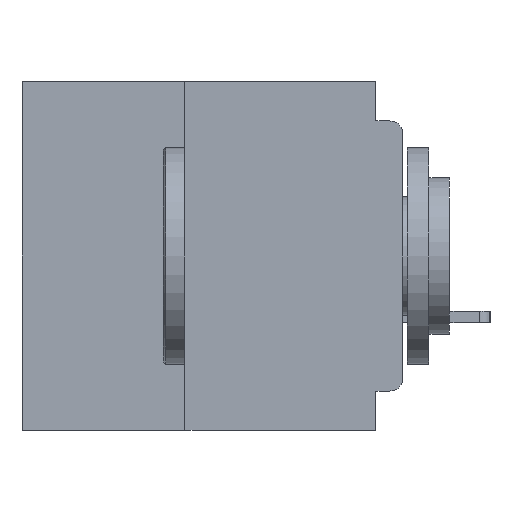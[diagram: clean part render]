
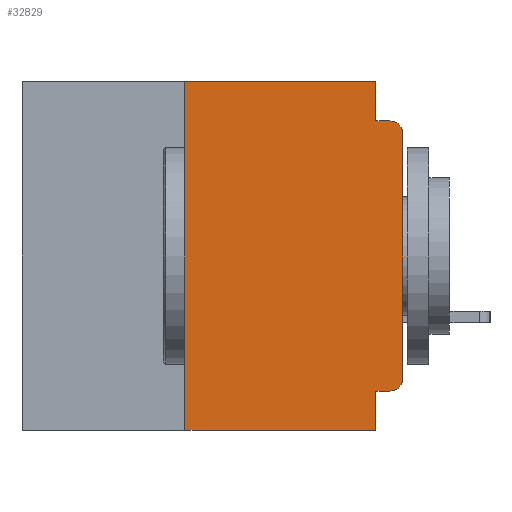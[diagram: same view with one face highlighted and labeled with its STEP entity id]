
A CAD part, left-side view. The second image highlights one B-rep face of the part: STEP entity #32829.
In plain terms, the highlighted planar face has unit normal (-1, 0, 0).
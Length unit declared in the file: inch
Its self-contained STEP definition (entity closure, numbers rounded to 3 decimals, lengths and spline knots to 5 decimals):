
#755 = EDGE_CURVE ( 'NONE', #26749, #22927, #27107, .T. ) ;
#1217 = VERTEX_POINT ( 'NONE', #17277 ) ;
#2097 = CARTESIAN_POINT ( 'NONE',  ( 0., 0.25, -0.4 ) ) ;
#2519 = LINE ( 'NONE', #15408, #29852 ) ;
#2727 = EDGE_CURVE ( 'NONE', #25477, #30640, #42923, .T. ) ;
#2748 = DIRECTION ( 'NONE',  ( 0., 0., -1. ) ) ;
#3197 = DIRECTION ( 'NONE',  ( 0., -1., 0. ) ) ;
#3625 = DIRECTION ( 'NONE',  ( 0., -1., 0. ) ) ;
#4621 = PLANE ( 'NONE',  #19149 ) ;
#4653 = LINE ( 'NONE', #6060, #37784 ) ;
#5015 = CARTESIAN_POINT ( 'NONE',  ( 0., 0.437, 0. ) ) ;
#5063 = DIRECTION ( 'NONE',  ( -1., 0., 0. ) ) ;
#6060 = CARTESIAN_POINT ( 'NONE',  ( 0., 0., 0. ) ) ;
#6274 = EDGE_CURVE ( 'NONE', #40019, #30336, #25094, .T. ) ;
#6362 = CARTESIAN_POINT ( 'NONE',  ( 0., 0.015, -0.355 ) ) ;
#6806 = EDGE_CURVE ( 'NONE', #17599, #1217, #4653, .T. ) ;
#6890 = VECTOR ( 'NONE', #3197, 39.37008 ) ;
#7023 = EDGE_CURVE ( 'NONE', #22927, #40019, #11173, .T. ) ;
#7667 = DIRECTION ( 'NONE',  ( 0., 1., 0. ) ) ;
#7726 = CARTESIAN_POINT ( 'NONE',  ( 0., 0., -0.355 ) ) ;
#9348 = FACE_OUTER_BOUND ( 'NONE', #37661, .T. ) ;
#9365 = ORIENTED_EDGE ( 'NONE', *, *, #25810, .T. ) ;
#10627 = EDGE_CURVE ( 'NONE', #10628, #26749, #10819, .T. ) ;
#10628 = VERTEX_POINT ( 'NONE', #39524 ) ;
#10819 = LINE ( 'NONE', #2097, #43734 ) ;
#10919 = CARTESIAN_POINT ( 'NONE',  ( 0., 0.031, 0. ) ) ;
#11173 = LINE ( 'NONE', #10919, #30289 ) ;
#11627 = DIRECTION ( 'NONE',  ( 0., 0., -1. ) ) ;
#12777 = AXIS2_PLACEMENT_3D ( 'NONE', #25591, #5063, #28982 ) ;
#13390 = VECTOR ( 'NONE', #2748, 39.37008 ) ;
#13480 = CARTESIAN_POINT ( 'NONE',  ( 0., 0.031, -0.045 ) ) ;
#14261 = EDGE_CURVE ( 'NONE', #30640, #40610, #30341, .T. ) ;
#15408 = CARTESIAN_POINT ( 'NONE',  ( 0., 0.437, -0.4 ) ) ;
#17057 = CARTESIAN_POINT ( 'NONE',  ( 0., 0.031, 0. ) ) ;
#17277 = CARTESIAN_POINT ( 'NONE',  ( 0., 0., -0.06 ) ) ;
#17599 = VERTEX_POINT ( 'NONE', #30851 ) ;
#18838 = DIRECTION ( 'NONE',  ( -1., 0., 0. ) ) ;
#19149 = AXIS2_PLACEMENT_3D ( 'NONE', #28546, #31941, #11627 ) ;
#21229 = ORIENTED_EDGE ( 'NONE', *, *, #29118, .T. ) ;
#22746 = ORIENTED_EDGE ( 'NONE', *, *, #14261, .F. ) ;
#22927 = VERTEX_POINT ( 'NONE', #17057 ) ;
#23232 = CARTESIAN_POINT ( 'NONE',  ( 0., 0.25, 0. ) ) ;
#23519 = CARTESIAN_POINT ( 'NONE',  ( 0., 0.031, -0.4 ) ) ;
#25030 = VECTOR ( 'NONE', #3625, 39.37008 ) ;
#25094 = LINE ( 'NONE', #44088, #6890 ) ;
#25477 = VERTEX_POINT ( 'NONE', #6362 ) ;
#25591 = CARTESIAN_POINT ( 'NONE',  ( 0., 0.015, -0.34 ) ) ;
#25810 = EDGE_CURVE ( 'NONE', #10628, #40610, #2519, .T. ) ;
#26414 = CIRCLE ( 'NONE', #12777, 0.015 ) ;
#26749 = VERTEX_POINT ( 'NONE', #23232 ) ;
#27107 = LINE ( 'NONE', #5015, #25030 ) ;
#28546 = CARTESIAN_POINT ( 'NONE',  ( 0., 0.437, 0. ) ) ;
#28982 = DIRECTION ( 'NONE',  ( 0., 0., -1. ) ) ;
#29118 = EDGE_CURVE ( 'NONE', #25477, #17599, #26414, .T. ) ;
#29380 = AXIS2_PLACEMENT_3D ( 'NONE', #39161, #18838, #42553 ) ;
#29445 = CARTESIAN_POINT ( 'NONE',  ( 0., 0.015, -0.045 ) ) ;
#29852 = VECTOR ( 'NONE', #39137, 39.37008 ) ;
#30289 = VECTOR ( 'NONE', #34673, 39.37008 ) ;
#30336 = VERTEX_POINT ( 'NONE', #29445 ) ;
#30341 = LINE ( 'NONE', #43654, #13390 ) ;
#30640 = VERTEX_POINT ( 'NONE', #40899 ) ;
#30851 = CARTESIAN_POINT ( 'NONE',  ( 0., 0., -0.34 ) ) ;
#31941 = DIRECTION ( 'NONE',  ( 1., 0., 0. ) ) ;
#32829 = ADVANCED_FACE ( 'NONE', ( #9348 ), #4621, .F. ) ;
#33253 = ORIENTED_EDGE ( 'NONE', *, *, #6806, .T. ) ;
#33495 = DIRECTION ( 'NONE',  ( 0., 0., 1. ) ) ;
#33870 = VECTOR ( 'NONE', #7667, 39.37008 ) ;
#34030 = EDGE_CURVE ( 'NONE', #1217, #30336, #38089, .T. ) ;
#34673 = DIRECTION ( 'NONE',  ( 0., 0., -1. ) ) ;
#34896 = ORIENTED_EDGE ( 'NONE', *, *, #755, .F. ) ;
#37565 = ORIENTED_EDGE ( 'NONE', *, *, #6274, .F. ) ;
#37661 = EDGE_LOOP ( 'NONE', ( #33253, #43360, #37565, #40770, #34896, #42366, #9365, #22746, #39237, #21229 ) ) ;
#37784 = VECTOR ( 'NONE', #33495, 39.37008 ) ;
#38089 = CIRCLE ( 'NONE', #29380, 0.015 ) ;
#39137 = DIRECTION ( 'NONE',  ( 0., -1., 0. ) ) ;
#39161 = CARTESIAN_POINT ( 'NONE',  ( 0., 0.015, -0.06 ) ) ;
#39237 = ORIENTED_EDGE ( 'NONE', *, *, #2727, .F. ) ;
#39524 = CARTESIAN_POINT ( 'NONE',  ( 0., 0.25, -0.4 ) ) ;
#39662 = DIRECTION ( 'NONE',  ( 0., 0., 1. ) ) ;
#40019 = VERTEX_POINT ( 'NONE', #13480 ) ;
#40610 = VERTEX_POINT ( 'NONE', #23519 ) ;
#40770 = ORIENTED_EDGE ( 'NONE', *, *, #7023, .F. ) ;
#40899 = CARTESIAN_POINT ( 'NONE',  ( 0., 0.031, -0.355 ) ) ;
#42366 = ORIENTED_EDGE ( 'NONE', *, *, #10627, .F. ) ;
#42553 = DIRECTION ( 'NONE',  ( 0., 0., -1. ) ) ;
#42923 = LINE ( 'NONE', #7726, #33870 ) ;
#43360 = ORIENTED_EDGE ( 'NONE', *, *, #34030, .T. ) ;
#43654 = CARTESIAN_POINT ( 'NONE',  ( 0., 0.031, -0.4 ) ) ;
#43734 = VECTOR ( 'NONE', #39662, 39.37008 ) ;
#44088 = CARTESIAN_POINT ( 'NONE',  ( 0., 0., -0.045 ) ) ;
